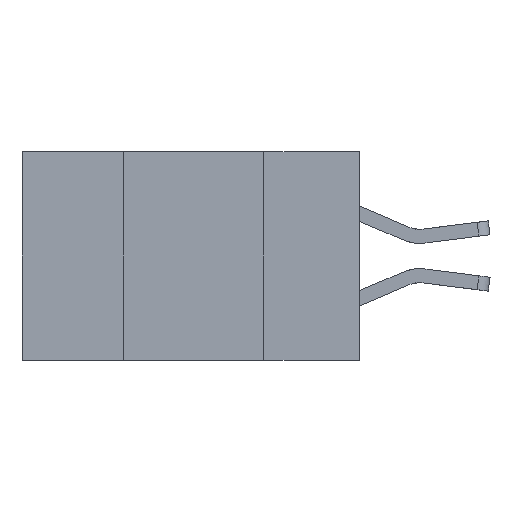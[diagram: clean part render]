
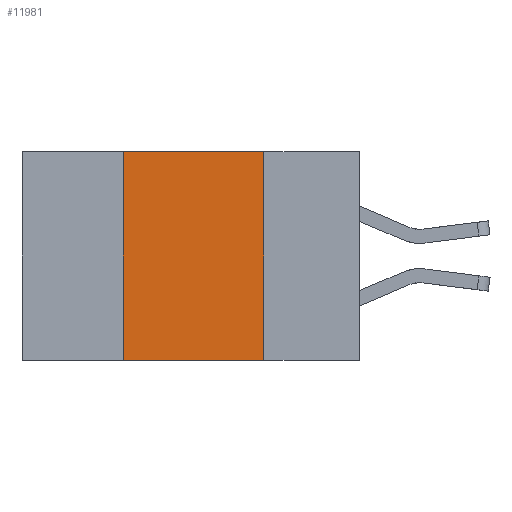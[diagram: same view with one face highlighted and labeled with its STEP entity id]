
A CAD part, left-side view. The second image highlights one B-rep face of the part: STEP entity #11981.
In plain terms, the highlighted planar face has unit normal (-1, 0, 0).
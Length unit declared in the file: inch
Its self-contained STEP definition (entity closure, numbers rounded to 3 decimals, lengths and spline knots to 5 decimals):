
#906 = VERTEX_POINT ( 'NONE', #5766 ) ;
#1543 = VECTOR ( 'NONE', #10737, 39.37008 ) ;
#2050 = EDGE_LOOP ( 'NONE', ( #2073, #2090, #2185, #2232 ) ) ;
#2073 = ORIENTED_EDGE ( 'NONE', *, *, #11001, .F. ) ;
#2090 = ORIENTED_EDGE ( 'NONE', *, *, #3030, .F. ) ;
#2099 = CARTESIAN_POINT ( 'NONE',  ( 0., 0.17, -0.37 ) ) ;
#2185 = ORIENTED_EDGE ( 'NONE', *, *, #13792, .F. ) ;
#2232 = ORIENTED_EDGE ( 'NONE', *, *, #6309, .T. ) ;
#2420 = VECTOR ( 'NONE', #4145, 39.37008 ) ;
#3030 = EDGE_CURVE ( 'NONE', #906, #11071, #7369, .T. ) ;
#4013 = CARTESIAN_POINT ( 'NONE',  ( 0., 0.42, -0.37 ) ) ;
#4145 = DIRECTION ( 'NONE',  ( 0., -1., 0. ) ) ;
#4251 = FACE_OUTER_BOUND ( 'NONE', #2050, .T. ) ;
#5766 = CARTESIAN_POINT ( 'NONE',  ( 0., 0.42, 0. ) ) ;
#6161 = VECTOR ( 'NONE', #13726, 39.37008 ) ;
#6178 = CARTESIAN_POINT ( 'NONE',  ( 0., 0.42, 0. ) ) ;
#6309 = EDGE_CURVE ( 'NONE', #13825, #7100, #8794, .T. ) ;
#6435 = CARTESIAN_POINT ( 'NONE',  ( 0., 0.6, 0. ) ) ;
#7100 = VERTEX_POINT ( 'NONE', #2099 ) ;
#7369 = LINE ( 'NONE', #7495, #1543 ) ;
#7495 = CARTESIAN_POINT ( 'NONE',  ( 0., 0.6, 0. ) ) ;
#7563 = DIRECTION ( 'NONE',  ( 0., 0., -1. ) ) ;
#8320 = CARTESIAN_POINT ( 'NONE',  ( 0., 0.17, 0. ) ) ;
#8439 = LINE ( 'NONE', #11475, #11319 ) ;
#8794 = LINE ( 'NONE', #11826, #2420 ) ;
#10040 = AXIS2_PLACEMENT_3D ( 'NONE', #6435, #13954, #7563 ) ;
#10737 = DIRECTION ( 'NONE',  ( 0., -1., 0. ) ) ;
#11001 = EDGE_CURVE ( 'NONE', #11071, #7100, #8439, .T. ) ;
#11071 = VERTEX_POINT ( 'NONE', #8320 ) ;
#11319 = VECTOR ( 'NONE', #12518, 39.37008 ) ;
#11475 = CARTESIAN_POINT ( 'NONE',  ( 0., 0.17, 0. ) ) ;
#11826 = CARTESIAN_POINT ( 'NONE',  ( 0., 0.6, -0.37 ) ) ;
#11949 = LINE ( 'NONE', #6178, #6161 ) ;
#11981 = ADVANCED_FACE ( 'NONE', ( #4251 ), #12901, .F. ) ;
#12518 = DIRECTION ( 'NONE',  ( 0., 0., -1. ) ) ;
#12901 = PLANE ( 'NONE',  #10040 ) ;
#13726 = DIRECTION ( 'NONE',  ( 0., 0., 1. ) ) ;
#13792 = EDGE_CURVE ( 'NONE', #13825, #906, #11949, .T. ) ;
#13825 = VERTEX_POINT ( 'NONE', #4013 ) ;
#13954 = DIRECTION ( 'NONE',  ( 1., 0., 0. ) ) ;
